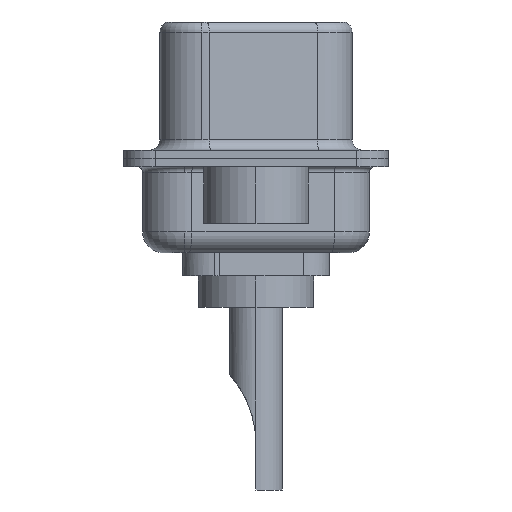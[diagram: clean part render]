
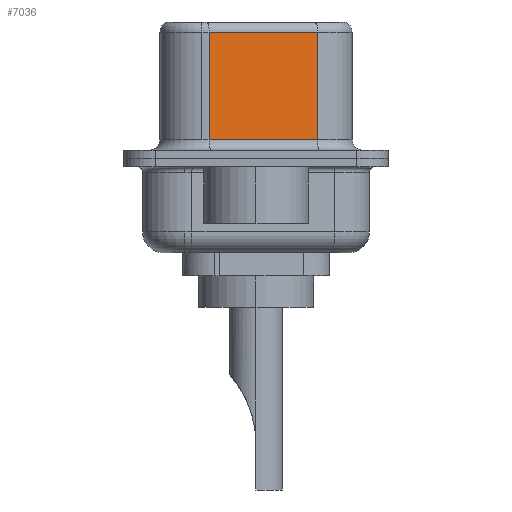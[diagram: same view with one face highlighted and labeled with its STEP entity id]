
A CAD part, left-side view. The second image highlights one B-rep face of the part: STEP entity #7036.
In plain terms, the highlighted planar face has unit normal (-0.985, -0.174, 0).
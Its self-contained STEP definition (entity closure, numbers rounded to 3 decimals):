
#389 = DIRECTION ( 'NONE',  ( 0.174, -0.985, 0. ) ) ;
#571 = ORIENTED_EDGE ( 'NONE', *, *, #9962, .T. ) ;
#808 = VECTOR ( 'NONE', #10825, 1000. ) ;
#1355 = VECTOR ( 'NONE', #389, 1000. ) ;
#1832 = VECTOR ( 'NONE', #7777, 1000. ) ;
#2732 = CARTESIAN_POINT ( 'NONE',  ( 3.675, 2.233, 0.9 ) ) ;
#2968 = VERTEX_POINT ( 'NONE', #2732 ) ;
#3165 = AXIS2_PLACEMENT_3D ( 'NONE', #14037, #5351, #14095 ) ;
#3726 = LINE ( 'NONE', #5209, #808 ) ;
#5209 = CARTESIAN_POINT ( 'NONE',  ( 4.585, -2.927, 6.52 ) ) ;
#5351 = DIRECTION ( 'NONE',  ( 0.985, 0.174, 0. ) ) ;
#5784 = DIRECTION ( 'NONE',  ( -0.174, 0.985, 0. ) ) ;
#5988 = CARTESIAN_POINT ( 'NONE',  ( 4.585, -2.927, 0.9 ) ) ;
#6389 = ORIENTED_EDGE ( 'NONE', *, *, #10169, .F. ) ;
#6658 = CARTESIAN_POINT ( 'NONE',  ( 3.675, 2.233, 6.52 ) ) ;
#6816 = VERTEX_POINT ( 'NONE', #5988 ) ;
#6971 = ORIENTED_EDGE ( 'NONE', *, *, #7535, .T. ) ;
#7036 = ADVANCED_FACE ( 'NONE', ( #7959 ), #9798, .F. ) ;
#7535 = EDGE_CURVE ( 'NONE', #7993, #2968, #10649, .T. ) ;
#7777 = DIRECTION ( 'NONE',  ( 0., 0., -1. ) ) ;
#7959 = FACE_OUTER_BOUND ( 'NONE', #11657, .T. ) ;
#7993 = VERTEX_POINT ( 'NONE', #13243 ) ;
#9798 = PLANE ( 'NONE',  #3165 ) ;
#9812 = LINE ( 'NONE', #13794, #1355 ) ;
#9962 = EDGE_CURVE ( 'NONE', #2968, #6816, #9812, .T. ) ;
#10169 = EDGE_CURVE ( 'NONE', #13183, #6816, #3726, .T. ) ;
#10453 = VECTOR ( 'NONE', #5784, 1000. ) ;
#10649 = LINE ( 'NONE', #6658, #1832 ) ;
#10817 = LINE ( 'NONE', #11436, #10453 ) ;
#10825 = DIRECTION ( 'NONE',  ( 0., 0., -1. ) ) ;
#11436 = CARTESIAN_POINT ( 'NONE',  ( 4.585, -2.927, 6.02 ) ) ;
#11657 = EDGE_LOOP ( 'NONE', ( #6389, #12709, #6971, #571 ) ) ;
#12166 = CARTESIAN_POINT ( 'NONE',  ( 4.585, -2.927, 6.02 ) ) ;
#12709 = ORIENTED_EDGE ( 'NONE', *, *, #13558, .T. ) ;
#13183 = VERTEX_POINT ( 'NONE', #12166 ) ;
#13243 = CARTESIAN_POINT ( 'NONE',  ( 3.675, 2.233, 6.02 ) ) ;
#13558 = EDGE_CURVE ( 'NONE', #13183, #7993, #10817, .T. ) ;
#13794 = CARTESIAN_POINT ( 'NONE',  ( 4.585, -2.927, 0.9 ) ) ;
#14037 = CARTESIAN_POINT ( 'NONE',  ( 4.585, -2.927, 6.52 ) ) ;
#14095 = DIRECTION ( 'NONE',  ( -0.174, 0.985, 0. ) ) ;
